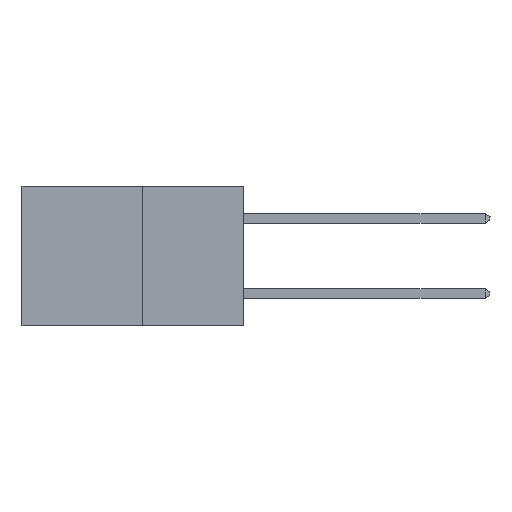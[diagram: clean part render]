
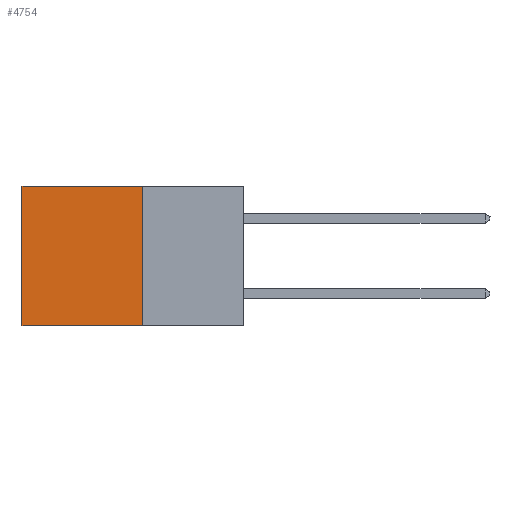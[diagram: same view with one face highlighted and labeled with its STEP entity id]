
A CAD part, left-side view. The second image highlights one B-rep face of the part: STEP entity #4754.
In plain terms, the highlighted planar face has unit normal (-1, 0, 0).
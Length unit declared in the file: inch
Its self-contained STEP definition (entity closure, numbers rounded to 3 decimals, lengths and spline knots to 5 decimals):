
#43 = EDGE_CURVE ( 'NONE', #9476, #215, #5110, .T. ) ;
#215 = VERTEX_POINT ( 'NONE', #9345 ) ;
#672 = CARTESIAN_POINT ( 'NONE',  ( 0.277, 0.27, 0. ) ) ;
#996 = ORIENTED_EDGE ( 'NONE', *, *, #43, .T. ) ;
#1016 = ORIENTED_EDGE ( 'NONE', *, *, #9303, .F. ) ;
#1284 = CARTESIAN_POINT ( 'NONE',  ( 0.277, 0.27, -0.37 ) ) ;
#1593 = VERTEX_POINT ( 'NONE', #5930 ) ;
#3068 = VECTOR ( 'NONE', #3517, 39.37008 ) ;
#3214 = PLANE ( 'NONE',  #9982 ) ;
#3517 = DIRECTION ( 'NONE',  ( 0., 1., 0. ) ) ;
#3932 = LINE ( 'NONE', #10094, #7513 ) ;
#4002 = CARTESIAN_POINT ( 'NONE',  ( 0.277, 0.27, -0.37 ) ) ;
#4165 = EDGE_LOOP ( 'NONE', ( #8756, #9864, #1016, #996 ) ) ;
#4523 = DIRECTION ( 'NONE',  ( 0., 1., 0. ) ) ;
#4754 = ADVANCED_FACE ( 'NONE', ( #10035 ), #3214, .F. ) ;
#4769 = DIRECTION ( 'NONE',  ( 1., 0., 0. ) ) ;
#4967 = VECTOR ( 'NONE', #8277, 39.37008 ) ;
#5110 = LINE ( 'NONE', #9832, #3068 ) ;
#5161 = DIRECTION ( 'NONE',  ( 0., 0., -1. ) ) ;
#5293 = CARTESIAN_POINT ( 'NONE',  ( 0.277, 0.27, -0.37 ) ) ;
#5930 = CARTESIAN_POINT ( 'NONE',  ( 0.277, 0.27, -0.37 ) ) ;
#5945 = LINE ( 'NONE', #5293, #9316 ) ;
#6249 = DIRECTION ( 'NONE',  ( 0., 0., -1. ) ) ;
#7485 = VERTEX_POINT ( 'NONE', #7601 ) ;
#7493 = LINE ( 'NONE', #1284, #4967 ) ;
#7513 = VECTOR ( 'NONE', #6249, 39.37008 ) ;
#7601 = CARTESIAN_POINT ( 'NONE',  ( 0.277, 0.59, -0.37 ) ) ;
#7688 = EDGE_CURVE ( 'NONE', #215, #7485, #3932, .T. ) ;
#8144 = EDGE_CURVE ( 'NONE', #1593, #7485, #5945, .T. ) ;
#8277 = DIRECTION ( 'NONE',  ( 0., 0., -1. ) ) ;
#8756 = ORIENTED_EDGE ( 'NONE', *, *, #7688, .T. ) ;
#9303 = EDGE_CURVE ( 'NONE', #9476, #1593, #7493, .T. ) ;
#9316 = VECTOR ( 'NONE', #4523, 39.37008 ) ;
#9345 = CARTESIAN_POINT ( 'NONE',  ( 0.277, 0.59, 0. ) ) ;
#9476 = VERTEX_POINT ( 'NONE', #672 ) ;
#9832 = CARTESIAN_POINT ( 'NONE',  ( 0.277, 0.27, 0. ) ) ;
#9864 = ORIENTED_EDGE ( 'NONE', *, *, #8144, .F. ) ;
#9982 = AXIS2_PLACEMENT_3D ( 'NONE', #4002, #4769, #5161 ) ;
#10035 = FACE_OUTER_BOUND ( 'NONE', #4165, .T. ) ;
#10094 = CARTESIAN_POINT ( 'NONE',  ( 0.277, 0.59, -0.37 ) ) ;
